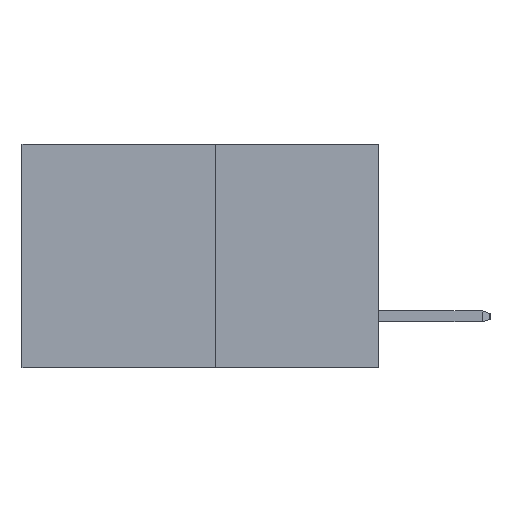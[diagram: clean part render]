
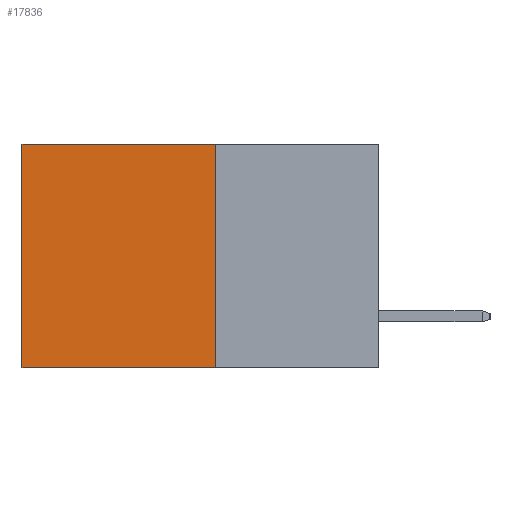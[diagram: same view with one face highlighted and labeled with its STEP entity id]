
A CAD part, left-side view. The second image highlights one B-rep face of the part: STEP entity #17836.
In plain terms, the highlighted planar face has unit normal (-1, 0, 0).
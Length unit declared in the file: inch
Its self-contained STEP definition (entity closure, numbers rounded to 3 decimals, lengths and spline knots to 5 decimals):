
#160 = VERTEX_POINT ( 'NONE', #13246 ) ;
#540 = CARTESIAN_POINT ( 'NONE',  ( 0.277, 0.27, -0.37 ) ) ;
#553 = VERTEX_POINT ( 'NONE', #19961 ) ;
#1807 = LINE ( 'NONE', #7959, #6006 ) ;
#2393 = DIRECTION ( 'NONE',  ( 1., 0., 0. ) ) ;
#3069 = CARTESIAN_POINT ( 'NONE',  ( 0.277, 0.59, 0. ) ) ;
#5739 = ORIENTED_EDGE ( 'NONE', *, *, #15145, .F. ) ;
#6006 = VECTOR ( 'NONE', #8394, 39.37008 ) ;
#6804 = DIRECTION ( 'NONE',  ( 0., 0., -1. ) ) ;
#7133 = EDGE_CURVE ( 'NONE', #160, #22160, #1807, .T. ) ;
#7559 = VECTOR ( 'NONE', #15796, 39.37008 ) ;
#7959 = CARTESIAN_POINT ( 'NONE',  ( 0.277, 0.27, 0. ) ) ;
#8394 = DIRECTION ( 'NONE',  ( 0., 1., 0. ) ) ;
#8618 = CARTESIAN_POINT ( 'NONE',  ( 0.277, 0.27, -0.37 ) ) ;
#9367 = VECTOR ( 'NONE', #16564, 39.37008 ) ;
#10510 = LINE ( 'NONE', #13942, #19474 ) ;
#11236 = CARTESIAN_POINT ( 'NONE',  ( 0.277, 0.27, -0.37 ) ) ;
#12304 = LINE ( 'NONE', #8618, #7559 ) ;
#12686 = ORIENTED_EDGE ( 'NONE', *, *, #7133, .T. ) ;
#13016 = FACE_OUTER_BOUND ( 'NONE', #19703, .T. ) ;
#13246 = CARTESIAN_POINT ( 'NONE',  ( 0.277, 0.27, 0. ) ) ;
#13564 = LINE ( 'NONE', #11236, #9367 ) ;
#13582 = CARTESIAN_POINT ( 'NONE',  ( 0.277, 0.27, -0.37 ) ) ;
#13942 = CARTESIAN_POINT ( 'NONE',  ( 0.277, 0.59, -0.37 ) ) ;
#14333 = VERTEX_POINT ( 'NONE', #13582 ) ;
#14921 = DIRECTION ( 'NONE',  ( 0., 0., -1. ) ) ;
#15145 = EDGE_CURVE ( 'NONE', #160, #14333, #12304, .T. ) ;
#15796 = DIRECTION ( 'NONE',  ( 0., 0., -1. ) ) ;
#16564 = DIRECTION ( 'NONE',  ( 0., 1., 0. ) ) ;
#16887 = EDGE_CURVE ( 'NONE', #22160, #553, #10510, .T. ) ;
#17823 = EDGE_CURVE ( 'NONE', #14333, #553, #13564, .T. ) ;
#17836 = ADVANCED_FACE ( 'NONE', ( #13016 ), #22038, .F. ) ;
#19474 = VECTOR ( 'NONE', #6804, 39.37008 ) ;
#19593 = ORIENTED_EDGE ( 'NONE', *, *, #16887, .T. ) ;
#19703 = EDGE_LOOP ( 'NONE', ( #19593, #21584, #5739, #12686 ) ) ;
#19961 = CARTESIAN_POINT ( 'NONE',  ( 0.277, 0.59, -0.37 ) ) ;
#21512 = AXIS2_PLACEMENT_3D ( 'NONE', #540, #2393, #14921 ) ;
#21584 = ORIENTED_EDGE ( 'NONE', *, *, #17823, .F. ) ;
#22038 = PLANE ( 'NONE',  #21512 ) ;
#22160 = VERTEX_POINT ( 'NONE', #3069 ) ;
